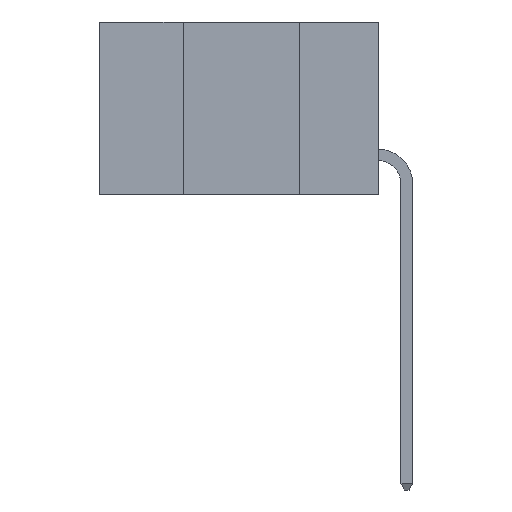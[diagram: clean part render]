
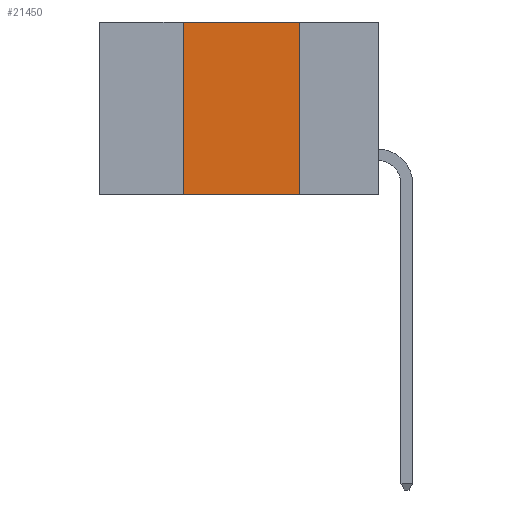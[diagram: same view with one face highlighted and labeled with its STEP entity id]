
A CAD part, left-side view. The second image highlights one B-rep face of the part: STEP entity #21450.
In plain terms, the highlighted planar face has unit normal (-1, 0, 0).
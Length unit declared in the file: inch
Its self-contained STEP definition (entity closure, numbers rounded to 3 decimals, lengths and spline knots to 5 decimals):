
#1008 = CARTESIAN_POINT ( 'NONE',  ( 0., 0.42, -0.37 ) ) ;
#1045 = CARTESIAN_POINT ( 'NONE',  ( 0., 0.17, -0.37 ) ) ;
#1159 = CARTESIAN_POINT ( 'NONE',  ( 0., 0.6, 0. ) ) ;
#1244 = CARTESIAN_POINT ( 'NONE',  ( 0., 0.17, 0. ) ) ;
#1555 = EDGE_CURVE ( 'NONE', #18290, #18947, #4389, .T. ) ;
#2104 = VECTOR ( 'NONE', #17913, 39.37008 ) ;
#2609 = DIRECTION ( 'NONE',  ( 0., 0., -1. ) ) ;
#4113 = ORIENTED_EDGE ( 'NONE', *, *, #1555, .T. ) ;
#4389 = LINE ( 'NONE', #6919, #6561 ) ;
#4616 = VERTEX_POINT ( 'NONE', #10555 ) ;
#4713 = FACE_OUTER_BOUND ( 'NONE', #13368, .T. ) ;
#5152 = VERTEX_POINT ( 'NONE', #1244 ) ;
#5629 = VECTOR ( 'NONE', #2609, 39.37008 ) ;
#6561 = VECTOR ( 'NONE', #21424, 39.37008 ) ;
#6919 = CARTESIAN_POINT ( 'NONE',  ( 0., 0.6, -0.37 ) ) ;
#7985 = DIRECTION ( 'NONE',  ( 0., 0., -1. ) ) ;
#8209 = AXIS2_PLACEMENT_3D ( 'NONE', #1159, #18140, #7985 ) ;
#8707 = VECTOR ( 'NONE', #16245, 39.37008 ) ;
#10218 = LINE ( 'NONE', #11186, #5629 ) ;
#10555 = CARTESIAN_POINT ( 'NONE',  ( 0., 0.42, 0. ) ) ;
#11186 = CARTESIAN_POINT ( 'NONE',  ( 0., 0.17, -0.37 ) ) ;
#11239 = LINE ( 'NONE', #16233, #2104 ) ;
#13318 = EDGE_CURVE ( 'NONE', #18290, #4616, #17734, .T. ) ;
#13368 = EDGE_LOOP ( 'NONE', ( #17292, #14787, #18190, #4113 ) ) ;
#14787 = ORIENTED_EDGE ( 'NONE', *, *, #16693, .F. ) ;
#15684 = CARTESIAN_POINT ( 'NONE',  ( 0., 0.42, -0.37 ) ) ;
#16233 = CARTESIAN_POINT ( 'NONE',  ( 0., 0.6, 0. ) ) ;
#16245 = DIRECTION ( 'NONE',  ( 0., 0., 1. ) ) ;
#16470 = PLANE ( 'NONE',  #8209 ) ;
#16693 = EDGE_CURVE ( 'NONE', #4616, #5152, #11239, .T. ) ;
#17292 = ORIENTED_EDGE ( 'NONE', *, *, #18921, .F. ) ;
#17734 = LINE ( 'NONE', #1008, #8707 ) ;
#17913 = DIRECTION ( 'NONE',  ( 0., -1., 0. ) ) ;
#18140 = DIRECTION ( 'NONE',  ( 1., 0., 0. ) ) ;
#18190 = ORIENTED_EDGE ( 'NONE', *, *, #13318, .F. ) ;
#18290 = VERTEX_POINT ( 'NONE', #15684 ) ;
#18921 = EDGE_CURVE ( 'NONE', #5152, #18947, #10218, .T. ) ;
#18947 = VERTEX_POINT ( 'NONE', #1045 ) ;
#21424 = DIRECTION ( 'NONE',  ( 0., -1., 0. ) ) ;
#21450 = ADVANCED_FACE ( 'NONE', ( #4713 ), #16470, .F. ) ;
